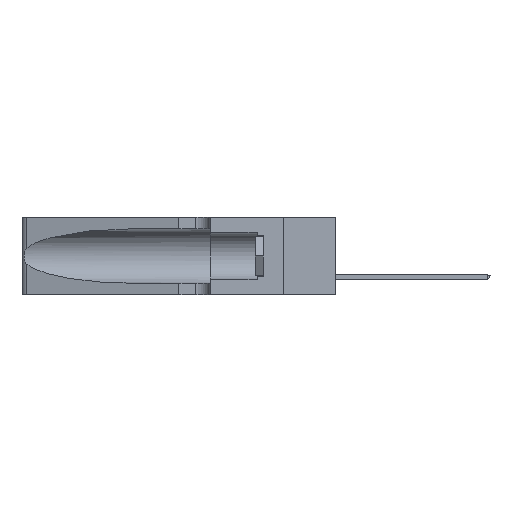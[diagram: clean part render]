
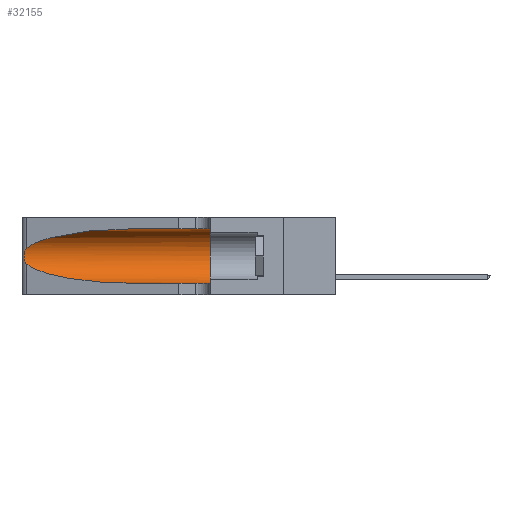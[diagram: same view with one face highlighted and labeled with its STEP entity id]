
A CAD part, left-side view. The second image highlights one B-rep face of the part: STEP entity #32155.
In plain terms, the highlighted cylindrical face has radius 3.308 mm (diameter 6.617 mm), a partial arc.
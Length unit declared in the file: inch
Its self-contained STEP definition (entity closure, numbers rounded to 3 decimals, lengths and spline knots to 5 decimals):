
#197 = CARTESIAN_POINT ( 'NONE',  ( 0.1305, 0.35, 0.31525 ) ) ;
#1330 = ORIENTED_EDGE ( 'NONE', *, *, #18723, .F. ) ;
#1425 = CARTESIAN_POINT ( 'NONE',  ( 0.1305, 0.35, 0.05475 ) ) ;
#2549 = CARTESIAN_POINT ( 'NONE',  ( 0.1305, 1.61858, 0.05475 ) ) ;
#3013 = EDGE_LOOP ( 'NONE', ( #37361, #5072, #22954, #22648, #48457, #1330 ) ) ;
#3617 =( BOUNDED_CURVE ( )  B_SPLINE_CURVE ( 3, ( #18571, #40666, #44662, #14648 ),
 .UNSPECIFIED., .F., .F. ) 
 B_SPLINE_CURVE_WITH_KNOTS ( ( 4, 4 ),
 ( 3.44316, 4.71239 ),
 .UNSPECIFIED. ) 
 CURVE ( )  GEOMETRIC_REPRESENTATION_ITEM ( )  RATIONAL_B_SPLINE_CURVE ( ( 1., 0.87, 0.87, 1. ) ) 
 REPRESENTATION_ITEM ( '' )  );
#4626 = CYLINDRICAL_SURFACE ( 'NONE', #40196, 0.13025 ) ;
#5072 = ORIENTED_EDGE ( 'NONE', *, *, #10418, .T. ) ;
#8803 = CARTESIAN_POINT ( 'NONE',  ( 0.1305, 1.61858, 0.185 ) ) ;
#9378 = CARTESIAN_POINT ( 'NONE',  ( 0.25555, 1.22993, 0.14849 ) ) ;
#9912 = CARTESIAN_POINT ( 'NONE',  ( 0.25789, 1.23486, 0.15765 ) ) ;
#10418 = EDGE_CURVE ( 'NONE', #17205, #32457, #39316, .T. ) ;
#10827 = CARTESIAN_POINT ( 'NONE',  ( 0.2373, 1.15595, 0.28018 ) ) ;
#11450 = CARTESIAN_POINT ( 'NONE',  ( 0.25487, 1.22718, 0.22369 ) ) ;
#11920 = AXIS2_PLACEMENT_3D ( 'NONE', #34797, #34970, #38925 ) ;
#14648 = CARTESIAN_POINT ( 'NONE',  ( 0.1305, 0.72297, 0.05475 ) ) ;
#16287 = CARTESIAN_POINT ( 'NONE',  ( 0.26075, 1.23896, 0.19203 ) ) ;
#17020 = EDGE_CURVE ( 'NONE', #42297, #17205, #30580, .T. ) ;
#17205 = VERTEX_POINT ( 'NONE', #47941 ) ;
#17616 = VECTOR ( 'NONE', #40793, 39.37008 ) ;
#18501 = EDGE_CURVE ( 'NONE', #48281, #25955, #21697, .T. ) ;
#18571 = CARTESIAN_POINT ( 'NONE',  ( 0.25487, 1.22718, 0.14631 ) ) ;
#18723 = EDGE_CURVE ( 'NONE', #42297, #48281, #24585, .T. ) ;
#19141 = CARTESIAN_POINT ( 'NONE',  ( 0.25639, 1.23184, 0.21858 ) ) ;
#19733 = CARTESIAN_POINT ( 'NONE',  ( 0.26018, 1.23835, 0.19895 ) ) ;
#20864 = CARTESIAN_POINT ( 'NONE',  ( 0.25487, 1.22718, 0.14631 ) ) ;
#21423 = CARTESIAN_POINT ( 'NONE',  ( 0.26075, 1.23896, 0.178 ) ) ;
#21580 = CARTESIAN_POINT ( 'NONE',  ( 0.1305, 0.72297, 0.05475 ) ) ;
#21697 = CIRCLE ( 'NONE', #11920, 0.13025 ) ;
#22470 = VERTEX_POINT ( 'NONE', #21580 ) ;
#22648 = ORIENTED_EDGE ( 'NONE', *, *, #25654, .T. ) ;
#22954 = ORIENTED_EDGE ( 'NONE', *, *, #47660, .T. ) ;
#24585 = LINE ( 'NONE', #36919, #46549 ) ;
#25252 = CARTESIAN_POINT ( 'NONE',  ( 0.25856, 1.23593, 0.16098 ) ) ;
#25300 = DIRECTION ( 'NONE',  ( 0., -1., 0. ) ) ;
#25353 = FACE_OUTER_BOUND ( 'NONE', #3013, .T. ) ;
#25654 = EDGE_CURVE ( 'NONE', #22470, #25955, #27615, .T. ) ;
#25716 = CARTESIAN_POINT ( 'NONE',  ( 0.25555, 1.22994, 0.2215 ) ) ;
#25955 = VERTEX_POINT ( 'NONE', #1425 ) ;
#27615 = LINE ( 'NONE', #2549, #17616 ) ;
#28078 = CARTESIAN_POINT ( 'NONE',  ( 0.25787, 1.23484, 0.2124 ) ) ;
#30511 = CARTESIAN_POINT ( 'NONE',  ( 0.1305, 0.72297, 0.31525 ) ) ;
#30580 =( BOUNDED_CURVE ( )  B_SPLINE_CURVE ( 3, ( #48041, #48885, #10827, #11450 ),
 .UNSPECIFIED., .F., .F. ) 
 B_SPLINE_CURVE_WITH_KNOTS ( ( 4, 4 ),
 ( 1.5708, 2.84003 ),
 .UNSPECIFIED. ) 
 CURVE ( )  GEOMETRIC_REPRESENTATION_ITEM ( )  RATIONAL_B_SPLINE_CURVE ( ( 1., 0.87, 0.87, 1. ) ) 
 REPRESENTATION_ITEM ( '' )  );
#32047 = CARTESIAN_POINT ( 'NONE',  ( 0.25639, 1.23186, 0.15144 ) ) ;
#32155 = ADVANCED_FACE ( 'NONE', ( #25353 ), #4626, .F. ) ;
#32457 = VERTEX_POINT ( 'NONE', #20864 ) ;
#34760 = DIRECTION ( 'NONE',  ( 0., -1., 0. ) ) ;
#34797 = CARTESIAN_POINT ( 'NONE',  ( 0.1305, 0.35, 0.185 ) ) ;
#34970 = DIRECTION ( 'NONE',  ( 0., 1., 0. ) ) ;
#35814 = CARTESIAN_POINT ( 'NONE',  ( 0.25487, 1.22718, 0.14631 ) ) ;
#36919 = CARTESIAN_POINT ( 'NONE',  ( 0.1305, 1.61858, 0.31525 ) ) ;
#37361 = ORIENTED_EDGE ( 'NONE', *, *, #17020, .T. ) ;
#38925 = DIRECTION ( 'NONE',  ( 0., 0., 1. ) ) ;
#39316 = B_SPLINE_CURVE_WITH_KNOTS ( 'NONE', 3,
 ( #41520, #25716, #19141, #28078, #40249, #19733, #16287, #21423, #47972, #25252, #9912, #32047, #9378, #35814 ),
 .UNSPECIFIED., .F., .F.,
 ( 4, 2, 2, 2, 2, 2, 4 ),
 ( 0., 0.00027, 0.00053, 0.00107, 0.0016, 0.00187, 0.00214 ),
 .UNSPECIFIED. ) ;
#40079 = DIRECTION ( 'NONE',  ( 0., 0., -1. ) ) ;
#40196 = AXIS2_PLACEMENT_3D ( 'NONE', #8803, #34760, #40079 ) ;
#40249 = CARTESIAN_POINT ( 'NONE',  ( 0.25854, 1.2359, 0.20912 ) ) ;
#40666 = CARTESIAN_POINT ( 'NONE',  ( 0.2373, 1.15595, 0.08982 ) ) ;
#40793 = DIRECTION ( 'NONE',  ( 0., -1., 0. ) ) ;
#41520 = CARTESIAN_POINT ( 'NONE',  ( 0.25487, 1.22718, 0.22369 ) ) ;
#42297 = VERTEX_POINT ( 'NONE', #30511 ) ;
#44662 = CARTESIAN_POINT ( 'NONE',  ( 0.18966, 0.96281, 0.05475 ) ) ;
#46549 = VECTOR ( 'NONE', #25300, 39.37008 ) ;
#47660 = EDGE_CURVE ( 'NONE', #32457, #22470, #3617, .T. ) ;
#47941 = CARTESIAN_POINT ( 'NONE',  ( 0.25487, 1.22718, 0.22369 ) ) ;
#47972 = CARTESIAN_POINT ( 'NONE',  ( 0.26017, 1.23833, 0.17102 ) ) ;
#48041 = CARTESIAN_POINT ( 'NONE',  ( 0.1305, 0.72297, 0.31525 ) ) ;
#48281 = VERTEX_POINT ( 'NONE', #197 ) ;
#48457 = ORIENTED_EDGE ( 'NONE', *, *, #18501, .F. ) ;
#48885 = CARTESIAN_POINT ( 'NONE',  ( 0.18966, 0.96281, 0.31525 ) ) ;
